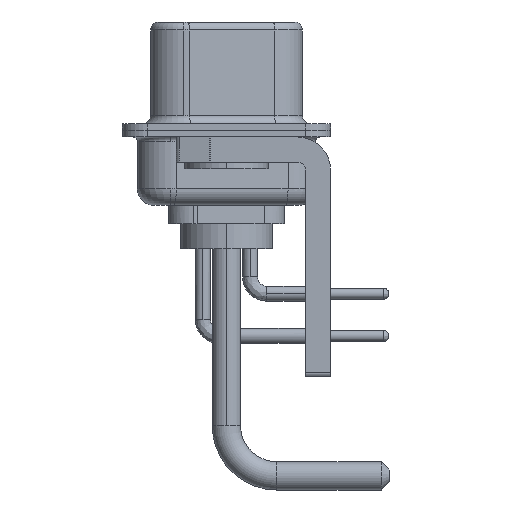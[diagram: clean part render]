
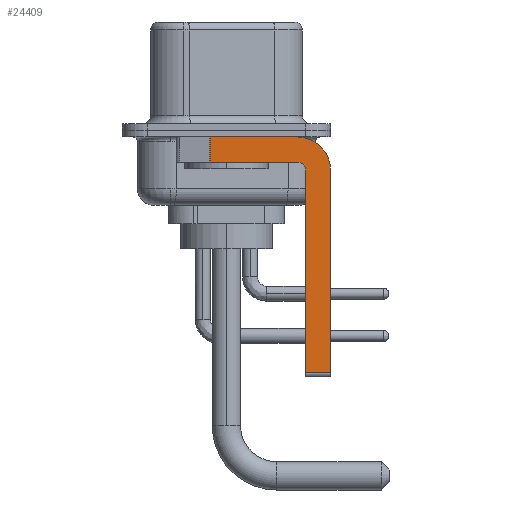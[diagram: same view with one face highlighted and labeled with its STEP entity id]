
A CAD part, left-side view. The second image highlights one B-rep face of the part: STEP entity #24409.
In plain terms, the highlighted planar face has unit normal (-1, 0, 0).
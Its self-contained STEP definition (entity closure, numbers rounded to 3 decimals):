
#38 = AXIS2_PLACEMENT_3D ( 'NONE', #27736, #3219, #10172 ) ;
#123 = LINE ( 'NONE', #8982, #13942 ) ;
#359 = ORIENTED_EDGE ( 'NONE', *, *, #11890, .F. ) ;
#1716 = VERTEX_POINT ( 'NONE', #26867 ) ;
#2302 = VECTOR ( 'NONE', #10215, 1000. ) ;
#3219 = DIRECTION ( 'NONE',  ( -1., 0., 0. ) ) ;
#3403 = VERTEX_POINT ( 'NONE', #13138 ) ;
#4115 = CIRCLE ( 'NONE', #20339, 2. ) ;
#4175 = DIRECTION ( 'NONE',  ( 0., 1., 0. ) ) ;
#4460 = ORIENTED_EDGE ( 'NONE', *, *, #24866, .F. ) ;
#4916 = DIRECTION ( 'NONE',  ( 0., -1., 0. ) ) ;
#5064 = VECTOR ( 'NONE', #28067, 1000. ) ;
#5356 = CARTESIAN_POINT ( 'NONE',  ( -2.9, -4.25, -2.4 ) ) ;
#5783 = DIRECTION ( 'NONE',  ( 0., 0., -1. ) ) ;
#6231 = VECTOR ( 'NONE', #16209, 1000. ) ;
#6935 = ORIENTED_EDGE ( 'NONE', *, *, #18728, .F. ) ;
#7370 = CARTESIAN_POINT ( 'NONE',  ( -2.9, 3., -0.4 ) ) ;
#7833 = CARTESIAN_POINT ( 'NONE',  ( -2.9, -4.25, -2.4 ) ) ;
#7946 = LINE ( 'NONE', #23884, #20291 ) ;
#8982 = CARTESIAN_POINT ( 'NONE',  ( -2.9, -4.25, -14.55 ) ) ;
#9010 = AXIS2_PLACEMENT_3D ( 'NONE', #5356, #16520, #19134 ) ;
#10172 = DIRECTION ( 'NONE',  ( 0., 0., 1. ) ) ;
#10215 = DIRECTION ( 'NONE',  ( 0., 0., 1. ) ) ;
#10350 = CARTESIAN_POINT ( 'NONE',  ( -2.9, -6.25, -2.4 ) ) ;
#10741 = DIRECTION ( 'NONE',  ( 0., 0., -1. ) ) ;
#10855 = EDGE_CURVE ( 'NONE', #1716, #28240, #21272, .T. ) ;
#11107 = ORIENTED_EDGE ( 'NONE', *, *, #11573, .T. ) ;
#11573 = EDGE_CURVE ( 'NONE', #1716, #20035, #123, .T. ) ;
#11770 = ORIENTED_EDGE ( 'NONE', *, *, #20869, .F. ) ;
#11890 = EDGE_CURVE ( 'NONE', #28240, #3403, #22760, .T. ) ;
#12550 = LINE ( 'NONE', #10350, #5064 ) ;
#12910 = CARTESIAN_POINT ( 'NONE',  ( -2.9, -6.25, -14.55 ) ) ;
#13113 = ORIENTED_EDGE ( 'NONE', *, *, #13209, .T. ) ;
#13128 = ORIENTED_EDGE ( 'NONE', *, *, #10855, .F. ) ;
#13138 = CARTESIAN_POINT ( 'NONE',  ( -2.9, -4.25, -1.9 ) ) ;
#13209 = EDGE_CURVE ( 'NONE', #19841, #28370, #23674, .T. ) ;
#13942 = VECTOR ( 'NONE', #4916, 1000. ) ;
#14420 = CARTESIAN_POINT ( 'NONE',  ( -2.9, -4.75, -14.8 ) ) ;
#16209 = DIRECTION ( 'NONE',  ( 0., -1., 0. ) ) ;
#16520 = DIRECTION ( 'NONE',  ( 1., 0., 0. ) ) ;
#16721 = EDGE_CURVE ( 'NONE', #3403, #28370, #7946, .T. ) ;
#17495 = CARTESIAN_POINT ( 'NONE',  ( -2.9, -6.25, -2.4 ) ) ;
#18237 = CARTESIAN_POINT ( 'NONE',  ( -2.9, -4.25, -0.4 ) ) ;
#18728 = EDGE_CURVE ( 'NONE', #24665, #25479, #4115, .T. ) ;
#19134 = DIRECTION ( 'NONE',  ( 0., 0., -1. ) ) ;
#19841 = VERTEX_POINT ( 'NONE', #23649 ) ;
#20035 = VERTEX_POINT ( 'NONE', #12910 ) ;
#20291 = VECTOR ( 'NONE', #4175, 1000. ) ;
#20339 = AXIS2_PLACEMENT_3D ( 'NONE', #7833, #27539, #5783 ) ;
#20605 = CARTESIAN_POINT ( 'NONE',  ( -2.9, -4.75, -2.4 ) ) ;
#20869 = EDGE_CURVE ( 'NONE', #25479, #20035, #12550, .T. ) ;
#20897 = PLANE ( 'NONE',  #9010 ) ;
#20999 = LINE ( 'NONE', #7370, #6231 ) ;
#21025 = FACE_OUTER_BOUND ( 'NONE', #21548, .T. ) ;
#21272 = LINE ( 'NONE', #14420, #2302 ) ;
#21548 = EDGE_LOOP ( 'NONE', ( #4460, #13113, #27590, #359, #13128, #11107, #11770, #6935 ) ) ;
#21803 = CARTESIAN_POINT ( 'NONE',  ( -2.9, 0.978, -1.9 ) ) ;
#22760 = CIRCLE ( 'NONE', #38, 0.5 ) ;
#23649 = CARTESIAN_POINT ( 'NONE',  ( -2.9, 0.978, -0.4 ) ) ;
#23674 = LINE ( 'NONE', #21803, #27114 ) ;
#23884 = CARTESIAN_POINT ( 'NONE',  ( -2.9, -4.25, -1.9 ) ) ;
#24409 = ADVANCED_FACE ( 'NONE', ( #21025 ), #20897, .F. ) ;
#24665 = VERTEX_POINT ( 'NONE', #18237 ) ;
#24866 = EDGE_CURVE ( 'NONE', #19841, #24665, #20999, .T. ) ;
#25479 = VERTEX_POINT ( 'NONE', #17495 ) ;
#25662 = CARTESIAN_POINT ( 'NONE',  ( -2.9, 0.978, -1.9 ) ) ;
#26867 = CARTESIAN_POINT ( 'NONE',  ( -2.9, -4.75, -14.55 ) ) ;
#27114 = VECTOR ( 'NONE', #10741, 1000. ) ;
#27539 = DIRECTION ( 'NONE',  ( 1., 0., 0. ) ) ;
#27590 = ORIENTED_EDGE ( 'NONE', *, *, #16721, .F. ) ;
#27736 = CARTESIAN_POINT ( 'NONE',  ( -2.9, -4.25, -2.4 ) ) ;
#28067 = DIRECTION ( 'NONE',  ( 0., 0., -1. ) ) ;
#28240 = VERTEX_POINT ( 'NONE', #20605 ) ;
#28370 = VERTEX_POINT ( 'NONE', #25662 ) ;
